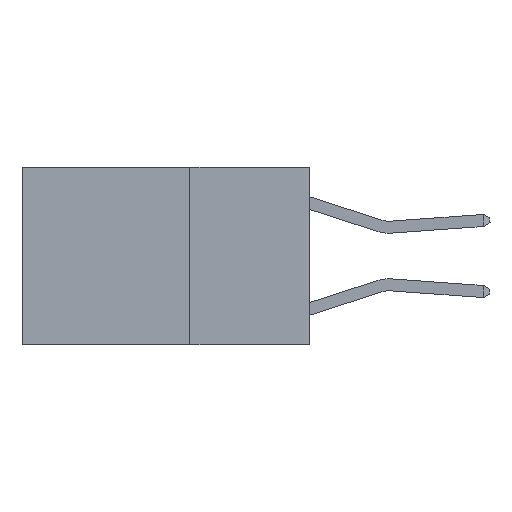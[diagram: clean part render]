
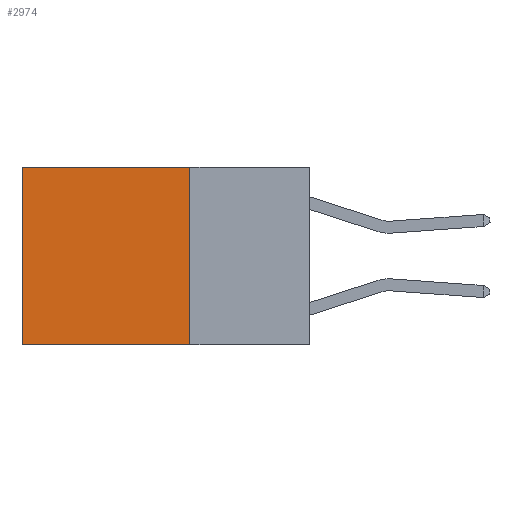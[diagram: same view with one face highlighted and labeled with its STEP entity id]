
A CAD part, left-side view. The second image highlights one B-rep face of the part: STEP entity #2974.
In plain terms, the highlighted planar face has unit normal (-1, 0, 0).
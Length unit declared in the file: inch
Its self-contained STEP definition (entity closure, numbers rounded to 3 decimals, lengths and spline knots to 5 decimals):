
#481 = EDGE_CURVE ( 'NONE', #9750, #10390, #1354, .T. ) ;
#1145 = ORIENTED_EDGE ( 'NONE', *, *, #8819, .F. ) ;
#1354 = LINE ( 'NONE', #1669, #3263 ) ;
#1418 = DIRECTION ( 'NONE',  ( 0., 1., 0. ) ) ;
#1424 = ORIENTED_EDGE ( 'NONE', *, *, #481, .T. ) ;
#1655 = LINE ( 'NONE', #7249, #9871 ) ;
#1669 = CARTESIAN_POINT ( 'NONE',  ( 0.2625, 0.25, 0. ) ) ;
#2013 = EDGE_CURVE ( 'NONE', #10390, #2363, #9352, .T. ) ;
#2363 = VERTEX_POINT ( 'NONE', #5355 ) ;
#2628 = CARTESIAN_POINT ( 'NONE',  ( 0.2625, 0.6, 0. ) ) ;
#2726 = FACE_OUTER_BOUND ( 'NONE', #9380, .T. ) ;
#2896 = PLANE ( 'NONE',  #6632 ) ;
#2974 = ADVANCED_FACE ( 'NONE', ( #2726 ), #2896, .F. ) ;
#3263 = VECTOR ( 'NONE', #1418, 39.37008 ) ;
#3705 = DIRECTION ( 'NONE',  ( 1., 0., 0. ) ) ;
#4508 = CARTESIAN_POINT ( 'NONE',  ( 0.2625, 0.25, 0. ) ) ;
#4838 = DIRECTION ( 'NONE',  ( 0., 0., -1. ) ) ;
#5307 = VECTOR ( 'NONE', #4838, 39.37008 ) ;
#5355 = CARTESIAN_POINT ( 'NONE',  ( 0.2625, 0.6, -0.37 ) ) ;
#5478 = ORIENTED_EDGE ( 'NONE', *, *, #6881, .F. ) ;
#6362 = CARTESIAN_POINT ( 'NONE',  ( 0.2625, 0.25, -0.37 ) ) ;
#6473 = CARTESIAN_POINT ( 'NONE',  ( 0.2625, 0.6, 0. ) ) ;
#6632 = AXIS2_PLACEMENT_3D ( 'NONE', #6902, #3705, #9263 ) ;
#6881 = EDGE_CURVE ( 'NONE', #9750, #8737, #9490, .T. ) ;
#6902 = CARTESIAN_POINT ( 'NONE',  ( 0.2625, 0.25, 0. ) ) ;
#7249 = CARTESIAN_POINT ( 'NONE',  ( 0.2625, 0.25, -0.37 ) ) ;
#7331 = ORIENTED_EDGE ( 'NONE', *, *, #2013, .T. ) ;
#7512 = VECTOR ( 'NONE', #8838, 39.37008 ) ;
#8737 = VERTEX_POINT ( 'NONE', #6362 ) ;
#8819 = EDGE_CURVE ( 'NONE', #8737, #2363, #1655, .T. ) ;
#8827 = DIRECTION ( 'NONE',  ( 0., 1., 0. ) ) ;
#8838 = DIRECTION ( 'NONE',  ( 0., 0., -1. ) ) ;
#9263 = DIRECTION ( 'NONE',  ( 0., 0., -1. ) ) ;
#9352 = LINE ( 'NONE', #6473, #7512 ) ;
#9380 = EDGE_LOOP ( 'NONE', ( #7331, #1145, #5478, #1424 ) ) ;
#9490 = LINE ( 'NONE', #10334, #5307 ) ;
#9750 = VERTEX_POINT ( 'NONE', #4508 ) ;
#9871 = VECTOR ( 'NONE', #8827, 39.37008 ) ;
#10334 = CARTESIAN_POINT ( 'NONE',  ( 0.2625, 0.25, 0. ) ) ;
#10390 = VERTEX_POINT ( 'NONE', #2628 ) ;
